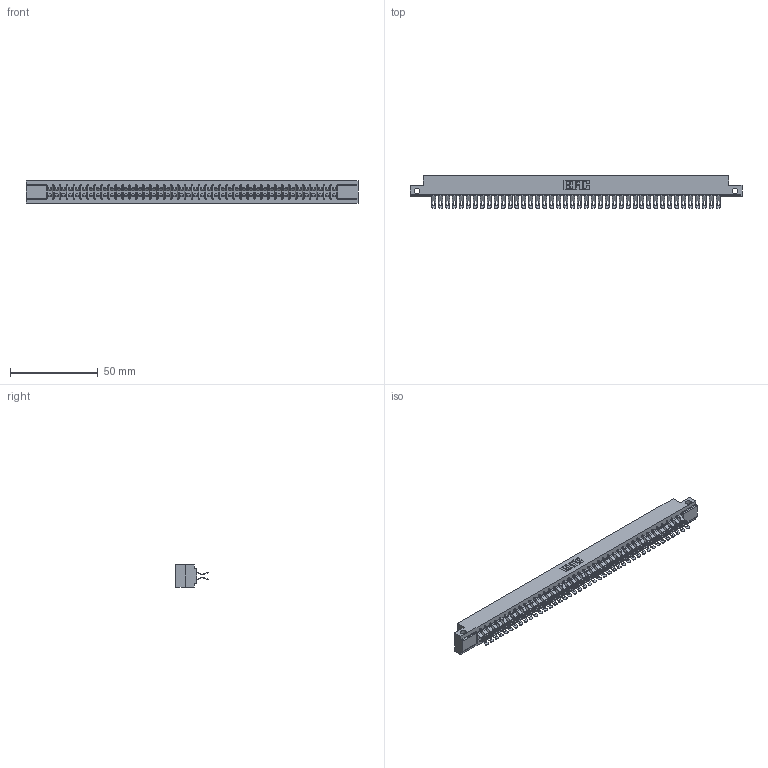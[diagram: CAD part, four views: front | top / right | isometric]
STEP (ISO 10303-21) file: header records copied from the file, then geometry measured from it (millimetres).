
FILE_DESCRIPTION (( 'STEP AP203' ), '1' );
FILE_NAME ('807-084-555-212.STEP', '2021-07-20T18:58:25', ( '' ), ( '' ), 'SwSTEP 2.0', 'SolidWorks 2020', '' );
FILE_SCHEMA (( 'CONFIG_CONTROL_DESIGN' ));
Length unit declared in the file: inch
Products named in the file (3): 307-290-001_555; 807 Part_.128 Dia Side Mounting Holes; 807-084-555-212
Assembly tree (85 placements, depth 2):
  807-084-555-212
    807 Part_.128 Dia Side Mounting Holes
    307-290-001_555  x84
Bounding box: 189.43 x 18.75 x 12.7 mm (x, y, z)
Volume: 20252.1 mm3; surface area: 26154.2 mm2
Topology: 85 solids, 85 shells, 5285 faces, 15527 edges, 10122 vertices
Faces by surface type: plane 2926, cylinder 2273, sphere 86
Entity records: 37889 total; most frequent: CARTESIAN_POINT 6202, ORIENTED_EDGE 6148, DIRECTION 6082, EDGE_CURVE 3074, VECTOR 2346, LINE 2346, VERTEX_POINT 1988, AXIS2_PLACEMENT_3D 1868
